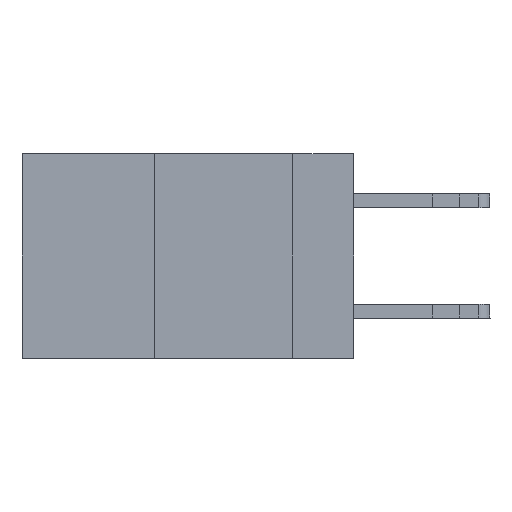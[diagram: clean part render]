
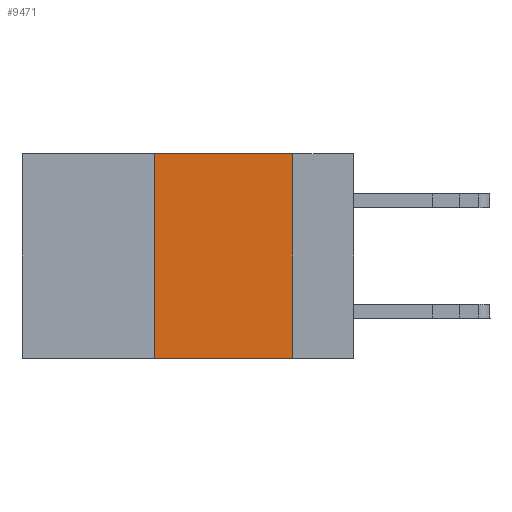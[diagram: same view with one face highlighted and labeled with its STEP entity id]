
A CAD part, left-side view. The second image highlights one B-rep face of the part: STEP entity #9471.
In plain terms, the highlighted planar face has unit normal (-1, 0, 0).
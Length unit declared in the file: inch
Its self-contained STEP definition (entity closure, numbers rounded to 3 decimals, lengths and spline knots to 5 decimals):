
#623 = CARTESIAN_POINT ( 'NONE',  ( 0., 0.36, -0.37 ) ) ;
#797 = AXIS2_PLACEMENT_3D ( 'NONE', #940, #14628, #4521 ) ;
#940 = CARTESIAN_POINT ( 'NONE',  ( 0., 0.6, 0. ) ) ;
#2193 = VECTOR ( 'NONE', #14369, 39.37008 ) ;
#2505 = CARTESIAN_POINT ( 'NONE',  ( 0., 0.6, 0. ) ) ;
#2826 = VERTEX_POINT ( 'NONE', #623 ) ;
#3156 = EDGE_CURVE ( 'NONE', #7944, #16957, #15311, .T. ) ;
#3613 = DIRECTION ( 'NONE',  ( 0., 0., -1. ) ) ;
#4521 = DIRECTION ( 'NONE',  ( 0., 0., -1. ) ) ;
#5464 = EDGE_CURVE ( 'NONE', #2826, #16646, #11795, .T. ) ;
#6211 = VECTOR ( 'NONE', #19352, 39.37008 ) ;
#6321 = CARTESIAN_POINT ( 'NONE',  ( 0., 0.36, 0. ) ) ;
#7699 = CARTESIAN_POINT ( 'NONE',  ( 0., 0.6, -0.37 ) ) ;
#7869 = ORIENTED_EDGE ( 'NONE', *, *, #12228, .F. ) ;
#7944 = VERTEX_POINT ( 'NONE', #10421 ) ;
#9176 = ORIENTED_EDGE ( 'NONE', *, *, #5464, .F. ) ;
#9471 = ADVANCED_FACE ( 'NONE', ( #19379 ), #12953, .F. ) ;
#10193 = LINE ( 'NONE', #7699, #6211 ) ;
#10421 = CARTESIAN_POINT ( 'NONE',  ( 0., 0.11, 0. ) ) ;
#10599 = DIRECTION ( 'NONE',  ( 0., 0., 1. ) ) ;
#10704 = LINE ( 'NONE', #2505, #2193 ) ;
#11795 = LINE ( 'NONE', #17187, #15740 ) ;
#12228 = EDGE_CURVE ( 'NONE', #16646, #7944, #10704, .T. ) ;
#12262 = EDGE_CURVE ( 'NONE', #2826, #16957, #10193, .T. ) ;
#12953 = PLANE ( 'NONE',  #797 ) ;
#13908 = CARTESIAN_POINT ( 'NONE',  ( 0., 0.11, -0.37 ) ) ;
#14369 = DIRECTION ( 'NONE',  ( 0., -1., 0. ) ) ;
#14554 = ORIENTED_EDGE ( 'NONE', *, *, #3156, .F. ) ;
#14628 = DIRECTION ( 'NONE',  ( 1., 0., 0. ) ) ;
#14747 = EDGE_LOOP ( 'NONE', ( #14554, #7869, #9176, #19649 ) ) ;
#15311 = LINE ( 'NONE', #17031, #19648 ) ;
#15740 = VECTOR ( 'NONE', #10599, 39.37008 ) ;
#16646 = VERTEX_POINT ( 'NONE', #6321 ) ;
#16957 = VERTEX_POINT ( 'NONE', #13908 ) ;
#17031 = CARTESIAN_POINT ( 'NONE',  ( 0., 0.11, 0. ) ) ;
#17187 = CARTESIAN_POINT ( 'NONE',  ( 0., 0.36, 0. ) ) ;
#19352 = DIRECTION ( 'NONE',  ( 0., -1., 0. ) ) ;
#19379 = FACE_OUTER_BOUND ( 'NONE', #14747, .T. ) ;
#19648 = VECTOR ( 'NONE', #3613, 39.37008 ) ;
#19649 = ORIENTED_EDGE ( 'NONE', *, *, #12262, .T. ) ;
